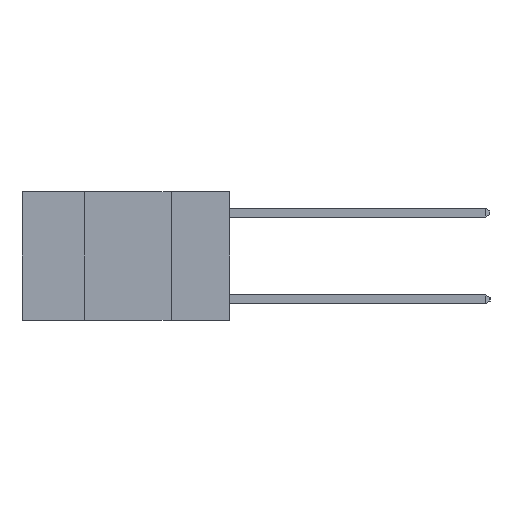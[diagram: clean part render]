
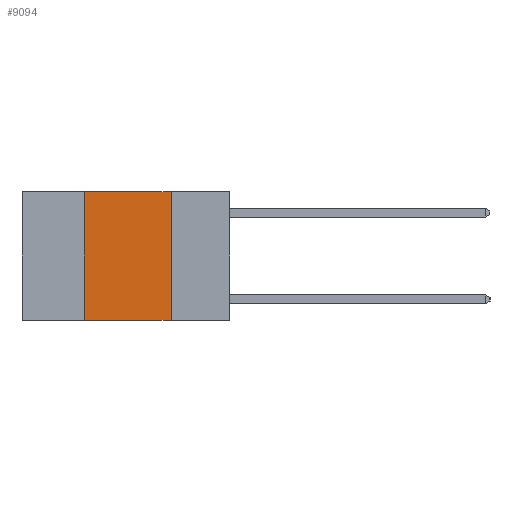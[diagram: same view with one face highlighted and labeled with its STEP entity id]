
A CAD part, left-side view. The second image highlights one B-rep face of the part: STEP entity #9094.
In plain terms, the highlighted planar face has unit normal (-1, 0, 0).
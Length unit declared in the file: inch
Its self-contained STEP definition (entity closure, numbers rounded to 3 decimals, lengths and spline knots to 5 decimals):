
#134 = CARTESIAN_POINT ( 'NONE',  ( 0., 0.6, 0. ) ) ;
#862 = VERTEX_POINT ( 'NONE', #7750 ) ;
#1054 = PLANE ( 'NONE',  #8808 ) ;
#1135 = EDGE_CURVE ( 'NONE', #8626, #9336, #6678, .T. ) ;
#1378 = EDGE_LOOP ( 'NONE', ( #9109, #8126, #3788, #3700 ) ) ;
#1663 = DIRECTION ( 'NONE',  ( 0., 0., -1. ) ) ;
#1817 = EDGE_CURVE ( 'NONE', #9336, #862, #6638, .T. ) ;
#2141 = CARTESIAN_POINT ( 'NONE',  ( 0., 0.6, -0.37 ) ) ;
#2918 = CARTESIAN_POINT ( 'NONE',  ( 0., 0.42, -0.37 ) ) ;
#2927 = LINE ( 'NONE', #2141, #4843 ) ;
#2984 = DIRECTION ( 'NONE',  ( 0., -1., 0. ) ) ;
#3596 = DIRECTION ( 'NONE',  ( 0., 0., -1. ) ) ;
#3700 = ORIENTED_EDGE ( 'NONE', *, *, #8199, .T. ) ;
#3788 = ORIENTED_EDGE ( 'NONE', *, *, #7930, .F. ) ;
#3792 = DIRECTION ( 'NONE',  ( 0., -1., 0. ) ) ;
#3873 = CARTESIAN_POINT ( 'NONE',  ( 0., 0.17, 0. ) ) ;
#4707 = VERTEX_POINT ( 'NONE', #2918 ) ;
#4732 = CARTESIAN_POINT ( 'NONE',  ( 0., 0.17, 0. ) ) ;
#4843 = VECTOR ( 'NONE', #2984, 39.37008 ) ;
#5893 = DIRECTION ( 'NONE',  ( 0., 0., 1. ) ) ;
#6638 = LINE ( 'NONE', #4732, #8614 ) ;
#6678 = LINE ( 'NONE', #8774, #10658 ) ;
#6778 = FACE_OUTER_BOUND ( 'NONE', #1378, .T. ) ;
#7734 = VECTOR ( 'NONE', #5893, 39.37008 ) ;
#7750 = CARTESIAN_POINT ( 'NONE',  ( 0., 0.17, -0.37 ) ) ;
#7930 = EDGE_CURVE ( 'NONE', #4707, #8626, #9821, .T. ) ;
#8126 = ORIENTED_EDGE ( 'NONE', *, *, #1135, .F. ) ;
#8199 = EDGE_CURVE ( 'NONE', #4707, #862, #2927, .T. ) ;
#8563 = DIRECTION ( 'NONE',  ( 1., 0., 0. ) ) ;
#8614 = VECTOR ( 'NONE', #1663, 39.37008 ) ;
#8626 = VERTEX_POINT ( 'NONE', #9993 ) ;
#8774 = CARTESIAN_POINT ( 'NONE',  ( 0., 0.6, 0. ) ) ;
#8808 = AXIS2_PLACEMENT_3D ( 'NONE', #134, #8563, #3596 ) ;
#9094 = ADVANCED_FACE ( 'NONE', ( #6778 ), #1054, .F. ) ;
#9109 = ORIENTED_EDGE ( 'NONE', *, *, #1817, .F. ) ;
#9336 = VERTEX_POINT ( 'NONE', #3873 ) ;
#9821 = LINE ( 'NONE', #10699, #7734 ) ;
#9993 = CARTESIAN_POINT ( 'NONE',  ( 0., 0.42, 0. ) ) ;
#10658 = VECTOR ( 'NONE', #3792, 39.37008 ) ;
#10699 = CARTESIAN_POINT ( 'NONE',  ( 0., 0.42, 0. ) ) ;
